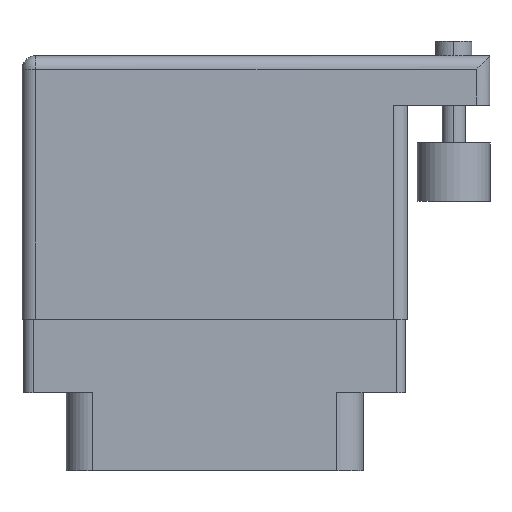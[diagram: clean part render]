
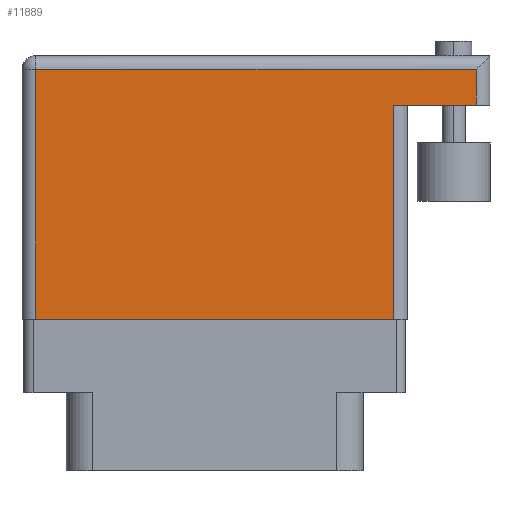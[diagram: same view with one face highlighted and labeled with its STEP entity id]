
A CAD part, front view. The second image highlights one B-rep face of the part: STEP entity #11889.
In plain terms, the highlighted face is planar.
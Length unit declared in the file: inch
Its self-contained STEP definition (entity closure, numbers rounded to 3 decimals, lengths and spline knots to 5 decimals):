
#1003 = DIRECTION ( 'NONE',  ( -1., 0., 0. ) ) ;
#1070 = CARTESIAN_POINT ( 'NONE',  ( 0.047, 0.859, 0. ) ) ;
#1376 = VERTEX_POINT ( 'NONE', #9249 ) ;
#1545 = DIRECTION ( 'NONE',  ( 0., -1., 0. ) ) ;
#1638 = DIRECTION ( 'NONE',  ( 0., 1., 0. ) ) ;
#2779 = DIRECTION ( 'NONE',  ( 0., 0., -1. ) ) ;
#2856 = EDGE_LOOP ( 'NONE', ( #16469, #25359, #15046, #22294, #25319, #6033 ) ) ;
#3072 = CARTESIAN_POINT ( 'NONE',  ( 0.047, 0., 0. ) ) ;
#3949 = VECTOR ( 'NONE', #1003, 39.37008 ) ;
#4114 = EDGE_CURVE ( 'NONE', #14044, #25527, #9818, .T. ) ;
#4737 = CARTESIAN_POINT ( 'NONE',  ( 1.278, 0., 0. ) ) ;
#4891 = CARTESIAN_POINT ( 'NONE',  ( 1.609, 0.736, 0. ) ) ;
#4970 = CARTESIAN_POINT ( 'NONE',  ( 0., 0.906, 0. ) ) ;
#5351 = CARTESIAN_POINT ( 'NONE',  ( 0.047, 0., 0. ) ) ;
#6033 = ORIENTED_EDGE ( 'NONE', *, *, #4114, .T. ) ;
#6391 = EDGE_CURVE ( 'NONE', #20059, #1376, #12933, .T. ) ;
#7030 = LINE ( 'NONE', #16818, #9930 ) ;
#7415 = AXIS2_PLACEMENT_3D ( 'NONE', #4970, #2779, #25641 ) ;
#9186 = VERTEX_POINT ( 'NONE', #18979 ) ;
#9249 = CARTESIAN_POINT ( 'NONE',  ( 1.278, 0.736, 0. ) ) ;
#9470 = EDGE_CURVE ( 'NONE', #25411, #1376, #18584, .T. ) ;
#9818 = LINE ( 'NONE', #5351, #22002 ) ;
#9930 = VECTOR ( 'NONE', #12787, 39.37008 ) ;
#11391 = EDGE_CURVE ( 'NONE', #20059, #9186, #7030, .T. ) ;
#11889 = ADVANCED_FACE ( 'NONE', ( #23359 ), #17062, .F. ) ;
#12575 = VECTOR ( 'NONE', #12722, 39.37008 ) ;
#12722 = DIRECTION ( 'NONE',  ( -1., 0., 0. ) ) ;
#12787 = DIRECTION ( 'NONE',  ( 0., 1., 0. ) ) ;
#12933 = LINE ( 'NONE', #4891, #3949 ) ;
#13126 = VECTOR ( 'NONE', #1638, 39.37008 ) ;
#14044 = VERTEX_POINT ( 'NONE', #1070 ) ;
#15046 = ORIENTED_EDGE ( 'NONE', *, *, #6391, .F. ) ;
#15458 = DIRECTION ( 'NONE',  ( 1., 0., 0. ) ) ;
#16469 = ORIENTED_EDGE ( 'NONE', *, *, #18778, .T. ) ;
#16521 = LINE ( 'NONE', #21569, #17194 ) ;
#16818 = CARTESIAN_POINT ( 'NONE',  ( 1.562, 0.906, 0. ) ) ;
#17062 = PLANE ( 'NONE',  #7415 ) ;
#17194 = VECTOR ( 'NONE', #15458, 39.37008 ) ;
#17295 = CARTESIAN_POINT ( 'NONE',  ( 1.562, 0.736, 0. ) ) ;
#18584 = LINE ( 'NONE', #21927, #13126 ) ;
#18778 = EDGE_CURVE ( 'NONE', #25527, #25411, #16521, .T. ) ;
#18844 = CARTESIAN_POINT ( 'NONE',  ( 0., 0.859, 0. ) ) ;
#18979 = CARTESIAN_POINT ( 'NONE',  ( 1.562, 0.859, 0. ) ) ;
#20059 = VERTEX_POINT ( 'NONE', #17295 ) ;
#20899 = EDGE_CURVE ( 'NONE', #9186, #14044, #23492, .T. ) ;
#21569 = CARTESIAN_POINT ( 'NONE',  ( 0., 0., 0. ) ) ;
#21927 = CARTESIAN_POINT ( 'NONE',  ( 1.278, 0.736, 0. ) ) ;
#22002 = VECTOR ( 'NONE', #1545, 39.37008 ) ;
#22294 = ORIENTED_EDGE ( 'NONE', *, *, #11391, .T. ) ;
#23359 = FACE_OUTER_BOUND ( 'NONE', #2856, .T. ) ;
#23492 = LINE ( 'NONE', #18844, #12575 ) ;
#25319 = ORIENTED_EDGE ( 'NONE', *, *, #20899, .T. ) ;
#25359 = ORIENTED_EDGE ( 'NONE', *, *, #9470, .T. ) ;
#25411 = VERTEX_POINT ( 'NONE', #4737 ) ;
#25527 = VERTEX_POINT ( 'NONE', #3072 ) ;
#25641 = DIRECTION ( 'NONE',  ( -1., 0., 0. ) ) ;
